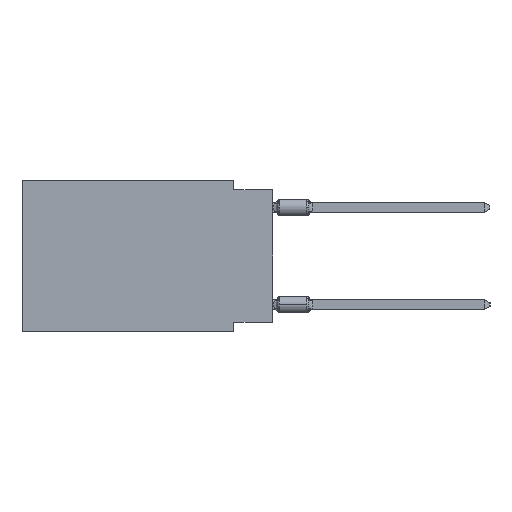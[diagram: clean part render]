
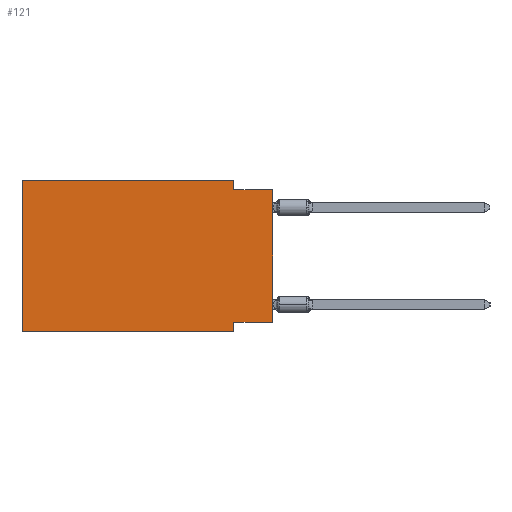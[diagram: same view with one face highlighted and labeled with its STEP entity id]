
A CAD part, left-side view. The second image highlights one B-rep face of the part: STEP entity #121.
In plain terms, the highlighted planar face has unit normal (-1, 0, 0).
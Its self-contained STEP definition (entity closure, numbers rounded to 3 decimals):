
#121 = ADVANCED_FACE ( 'NONE', ( #17206 ), #36303, .F. ) ;
#2837 = DIRECTION ( 'NONE',  ( 0., -1., 0. ) ) ;
#3615 = EDGE_LOOP ( 'NONE', ( #31189, #44278, #20818, #31020, #34969, #23840, #42667, #29637 ) ) ;
#5002 = VERTEX_POINT ( 'NONE', #8494 ) ;
#5079 = LINE ( 'NONE', #38614, #10047 ) ;
#7476 = DIRECTION ( 'NONE',  ( 0., 0., -1. ) ) ;
#8090 = LINE ( 'NONE', #56694, #36686 ) ;
#8494 = CARTESIAN_POINT ( 'NONE',  ( 0., 0., -9.271 ) ) ;
#8816 = DIRECTION ( 'NONE',  ( 0., 0., -1. ) ) ;
#10047 = VECTOR ( 'NONE', #19803, 1000. ) ;
#11666 = EDGE_CURVE ( 'NONE', #47461, #57382, #8090, .T. ) ;
#12184 = DIRECTION ( 'NONE',  ( 1., 0., 0. ) ) ;
#12703 = LINE ( 'NONE', #17716, #26330 ) ;
#13729 = DIRECTION ( 'NONE',  ( 0., 0., 1. ) ) ;
#14842 = CARTESIAN_POINT ( 'NONE',  ( 0., 0., -0.635 ) ) ;
#15686 = CARTESIAN_POINT ( 'NONE',  ( 0., 2.54, -9.271 ) ) ;
#15693 = CARTESIAN_POINT ( 'NONE',  ( 0., 2.54, 0. ) ) ;
#17206 = FACE_OUTER_BOUND ( 'NONE', #3615, .T. ) ;
#17613 = VERTEX_POINT ( 'NONE', #15686 ) ;
#17716 = CARTESIAN_POINT ( 'NONE',  ( 0., 2.54, 0. ) ) ;
#17994 = VECTOR ( 'NONE', #8816, 1000. ) ;
#19803 = DIRECTION ( 'NONE',  ( 0., 1., 0. ) ) ;
#20818 = ORIENTED_EDGE ( 'NONE', *, *, #30751, .F. ) ;
#20917 = LINE ( 'NONE', #45076, #30223 ) ;
#21271 = VECTOR ( 'NONE', #53811, 1000. ) ;
#21845 = DIRECTION ( 'NONE',  ( 0., -1., 0. ) ) ;
#22154 = CARTESIAN_POINT ( 'NONE',  ( 0., 0., -0.635 ) ) ;
#22728 = DIRECTION ( 'NONE',  ( 0., 0., -1. ) ) ;
#23140 = CARTESIAN_POINT ( 'NONE',  ( 0., 16.383, 0. ) ) ;
#23840 = ORIENTED_EDGE ( 'NONE', *, *, #30567, .T. ) ;
#25269 = EDGE_CURVE ( 'NONE', #17613, #38257, #51801, .T. ) ;
#26081 = EDGE_CURVE ( 'NONE', #5002, #17613, #5079, .T. ) ;
#26330 = VECTOR ( 'NONE', #22728, 1000. ) ;
#29372 = EDGE_CURVE ( 'NONE', #5002, #40633, #20917, .T. ) ;
#29637 = ORIENTED_EDGE ( 'NONE', *, *, #26081, .F. ) ;
#30223 = VECTOR ( 'NONE', #45388, 1000. ) ;
#30567 = EDGE_CURVE ( 'NONE', #47461, #38257, #49406, .T. ) ;
#30751 = EDGE_CURVE ( 'NONE', #56010, #36801, #12703, .T. ) ;
#31020 = ORIENTED_EDGE ( 'NONE', *, *, #32862, .F. ) ;
#31189 = ORIENTED_EDGE ( 'NONE', *, *, #29372, .T. ) ;
#32862 = EDGE_CURVE ( 'NONE', #57382, #56010, #36996, .T. ) ;
#34969 = ORIENTED_EDGE ( 'NONE', *, *, #11666, .F. ) ;
#36303 = PLANE ( 'NONE',  #61256 ) ;
#36686 = VECTOR ( 'NONE', #13729, 1000. ) ;
#36801 = VERTEX_POINT ( 'NONE', #44748 ) ;
#36996 = LINE ( 'NONE', #50513, #43524 ) ;
#37544 = EDGE_CURVE ( 'NONE', #36801, #40633, #59183, .T. ) ;
#38257 = VERTEX_POINT ( 'NONE', #53102 ) ;
#38614 = CARTESIAN_POINT ( 'NONE',  ( 0., 0., -9.271 ) ) ;
#40633 = VERTEX_POINT ( 'NONE', #14842 ) ;
#41906 = VECTOR ( 'NONE', #21845, 1000. ) ;
#42667 = ORIENTED_EDGE ( 'NONE', *, *, #25269, .F. ) ;
#43524 = VECTOR ( 'NONE', #2837, 1000. ) ;
#44278 = ORIENTED_EDGE ( 'NONE', *, *, #37544, .F. ) ;
#44748 = CARTESIAN_POINT ( 'NONE',  ( 0., 2.54, -0.635 ) ) ;
#45076 = CARTESIAN_POINT ( 'NONE',  ( 0., 0., 0. ) ) ;
#45388 = DIRECTION ( 'NONE',  ( 0., 0., 1. ) ) ;
#47461 = VERTEX_POINT ( 'NONE', #60895 ) ;
#48933 = CARTESIAN_POINT ( 'NONE',  ( 0., 16.383, 0. ) ) ;
#49406 = LINE ( 'NONE', #49721, #21271 ) ;
#49721 = CARTESIAN_POINT ( 'NONE',  ( 0., 16.383, -9.906 ) ) ;
#50513 = CARTESIAN_POINT ( 'NONE',  ( 0., 16.383, 0. ) ) ;
#51801 = LINE ( 'NONE', #55858, #17994 ) ;
#53102 = CARTESIAN_POINT ( 'NONE',  ( 0., 2.54, -9.906 ) ) ;
#53811 = DIRECTION ( 'NONE',  ( 0., -1., 0. ) ) ;
#55858 = CARTESIAN_POINT ( 'NONE',  ( 0., 2.54, -9.906 ) ) ;
#56010 = VERTEX_POINT ( 'NONE', #15693 ) ;
#56694 = CARTESIAN_POINT ( 'NONE',  ( 0., 16.383, 0. ) ) ;
#57382 = VERTEX_POINT ( 'NONE', #48933 ) ;
#59183 = LINE ( 'NONE', #22154, #41906 ) ;
#60895 = CARTESIAN_POINT ( 'NONE',  ( 0., 16.383, -9.906 ) ) ;
#61256 = AXIS2_PLACEMENT_3D ( 'NONE', #23140, #12184, #7476 ) ;
